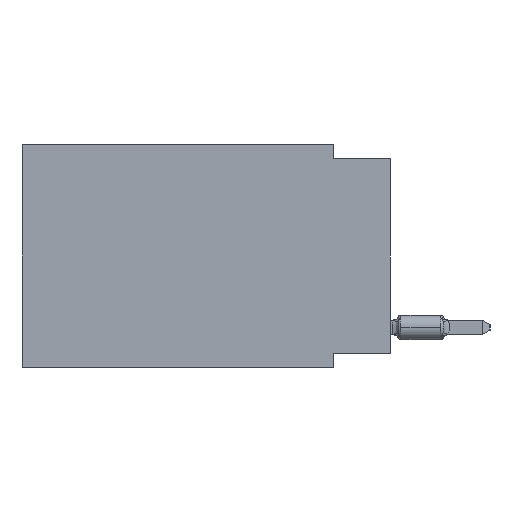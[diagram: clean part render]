
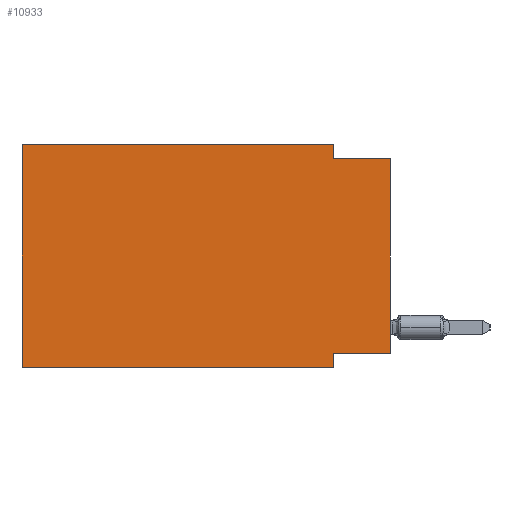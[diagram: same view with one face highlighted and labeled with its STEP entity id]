
A CAD part, left-side view. The second image highlights one B-rep face of the part: STEP entity #10933.
In plain terms, the highlighted planar face has unit normal (-1, 0, 0).
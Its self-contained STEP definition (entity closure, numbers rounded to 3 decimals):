
#148 = CARTESIAN_POINT ( 'NONE',  ( 0., 2.54, -9.271 ) ) ;
#1294 = VERTEX_POINT ( 'NONE', #14900 ) ;
#1617 = CARTESIAN_POINT ( 'NONE',  ( 0., 0., -0.635 ) ) ;
#1635 = CARTESIAN_POINT ( 'NONE',  ( 0., 0., 0. ) ) ;
#1898 = EDGE_LOOP ( 'NONE', ( #12534, #18201, #17849, #6831, #23705, #10973, #19585, #5207 ) ) ;
#2847 = CARTESIAN_POINT ( 'NONE',  ( 0., 16.383, 0. ) ) ;
#3722 = DIRECTION ( 'NONE',  ( 0., -1., 0. ) ) ;
#3853 = EDGE_CURVE ( 'NONE', #1294, #22762, #22782, .T. ) ;
#4293 = EDGE_CURVE ( 'NONE', #23144, #4914, #9768, .T. ) ;
#4765 = LINE ( 'NONE', #8345, #20770 ) ;
#4914 = VERTEX_POINT ( 'NONE', #22423 ) ;
#5207 = ORIENTED_EDGE ( 'NONE', *, *, #8226, .F. ) ;
#5582 = LINE ( 'NONE', #1635, #18151 ) ;
#5676 = VERTEX_POINT ( 'NONE', #148 ) ;
#6139 = VECTOR ( 'NONE', #20832, 1000. ) ;
#6785 = DIRECTION ( 'NONE',  ( 0., 0., -1. ) ) ;
#6817 = DIRECTION ( 'NONE',  ( 0., 0., -1. ) ) ;
#6831 = ORIENTED_EDGE ( 'NONE', *, *, #11296, .F. ) ;
#7840 = EDGE_CURVE ( 'NONE', #19413, #1294, #9735, .T. ) ;
#8226 = EDGE_CURVE ( 'NONE', #19625, #5676, #4765, .T. ) ;
#8345 = CARTESIAN_POINT ( 'NONE',  ( 0., 0., -9.271 ) ) ;
#9030 = VECTOR ( 'NONE', #3722, 1000. ) ;
#9735 = LINE ( 'NONE', #13699, #15001 ) ;
#9768 = LINE ( 'NONE', #13487, #6139 ) ;
#10269 = DIRECTION ( 'NONE',  ( 0., 1., 0. ) ) ;
#10933 = ADVANCED_FACE ( 'NONE', ( #23124 ), #22650, .F. ) ;
#10973 = ORIENTED_EDGE ( 'NONE', *, *, #15252, .T. ) ;
#11197 = DIRECTION ( 'NONE',  ( 0., -1., 0. ) ) ;
#11296 = EDGE_CURVE ( 'NONE', #4914, #19413, #19937, .T. ) ;
#12303 = LINE ( 'NONE', #15921, #17850 ) ;
#12534 = ORIENTED_EDGE ( 'NONE', *, *, #13292, .T. ) ;
#12675 = VERTEX_POINT ( 'NONE', #20444 ) ;
#13292 = EDGE_CURVE ( 'NONE', #19625, #22762, #5582, .T. ) ;
#13487 = CARTESIAN_POINT ( 'NONE',  ( 0., 16.383, 0. ) ) ;
#13645 = CARTESIAN_POINT ( 'NONE',  ( 0., 0., -0.635 ) ) ;
#13699 = CARTESIAN_POINT ( 'NONE',  ( 0., 2.54, 0. ) ) ;
#13824 = CARTESIAN_POINT ( 'NONE',  ( 0., 16.383, -9.906 ) ) ;
#14559 = VECTOR ( 'NONE', #20980, 1000. ) ;
#14900 = CARTESIAN_POINT ( 'NONE',  ( 0., 2.54, -0.635 ) ) ;
#15001 = VECTOR ( 'NONE', #6817, 1000. ) ;
#15252 = EDGE_CURVE ( 'NONE', #23144, #12675, #21906, .T. ) ;
#15921 = CARTESIAN_POINT ( 'NONE',  ( 0., 2.54, -9.906 ) ) ;
#15928 = AXIS2_PLACEMENT_3D ( 'NONE', #2847, #23000, #17138 ) ;
#17138 = DIRECTION ( 'NONE',  ( 0., 0., -1. ) ) ;
#17849 = ORIENTED_EDGE ( 'NONE', *, *, #7840, .F. ) ;
#17850 = VECTOR ( 'NONE', #6785, 1000. ) ;
#18078 = CARTESIAN_POINT ( 'NONE',  ( 0., 16.383, -9.906 ) ) ;
#18151 = VECTOR ( 'NONE', #20240, 1000. ) ;
#18201 = ORIENTED_EDGE ( 'NONE', *, *, #3853, .F. ) ;
#19267 = CARTESIAN_POINT ( 'NONE',  ( 0., 2.54, 0. ) ) ;
#19413 = VERTEX_POINT ( 'NONE', #19267 ) ;
#19585 = ORIENTED_EDGE ( 'NONE', *, *, #20811, .F. ) ;
#19625 = VERTEX_POINT ( 'NONE', #23575 ) ;
#19937 = LINE ( 'NONE', #20178, #9030 ) ;
#20178 = CARTESIAN_POINT ( 'NONE',  ( 0., 16.383, 0. ) ) ;
#20240 = DIRECTION ( 'NONE',  ( 0., 0., 1. ) ) ;
#20444 = CARTESIAN_POINT ( 'NONE',  ( 0., 2.54, -9.906 ) ) ;
#20770 = VECTOR ( 'NONE', #10269, 1000. ) ;
#20811 = EDGE_CURVE ( 'NONE', #5676, #12675, #12303, .T. ) ;
#20832 = DIRECTION ( 'NONE',  ( 0., 0., 1. ) ) ;
#20980 = DIRECTION ( 'NONE',  ( 0., -1., 0. ) ) ;
#21906 = LINE ( 'NONE', #18078, #23137 ) ;
#22423 = CARTESIAN_POINT ( 'NONE',  ( 0., 16.383, 0. ) ) ;
#22650 = PLANE ( 'NONE',  #15928 ) ;
#22762 = VERTEX_POINT ( 'NONE', #1617 ) ;
#22782 = LINE ( 'NONE', #13645, #14559 ) ;
#23000 = DIRECTION ( 'NONE',  ( 1., 0., 0. ) ) ;
#23124 = FACE_OUTER_BOUND ( 'NONE', #1898, .T. ) ;
#23137 = VECTOR ( 'NONE', #11197, 1000. ) ;
#23144 = VERTEX_POINT ( 'NONE', #13824 ) ;
#23575 = CARTESIAN_POINT ( 'NONE',  ( 0., 0., -9.271 ) ) ;
#23705 = ORIENTED_EDGE ( 'NONE', *, *, #4293, .F. ) ;
